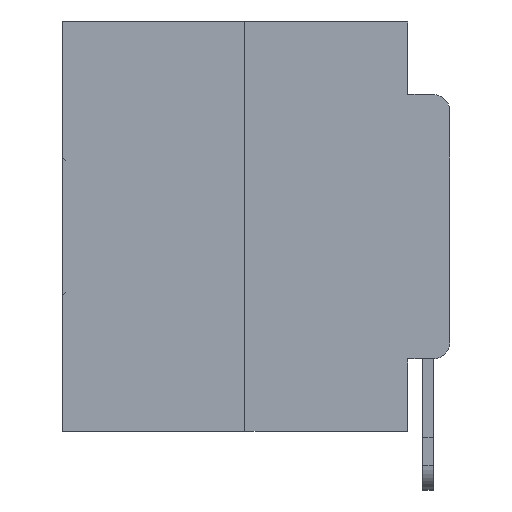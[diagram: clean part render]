
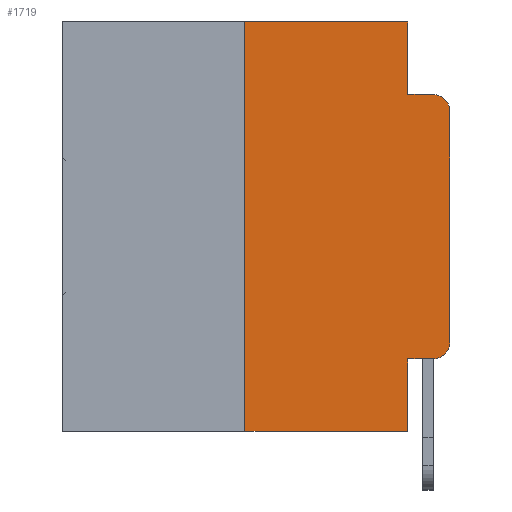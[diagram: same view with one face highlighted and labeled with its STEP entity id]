
A CAD part, left-side view. The second image highlights one B-rep face of the part: STEP entity #1719.
In plain terms, the highlighted planar face has unit normal (-1, 0, 0).
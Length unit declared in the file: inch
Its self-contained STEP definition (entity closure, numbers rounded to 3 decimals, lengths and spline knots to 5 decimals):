
#483 = VERTEX_POINT ( 'NONE', #22196 ) ;
#637 = EDGE_CURVE ( 'NONE', #29164, #14977, #27600, .T. ) ;
#1609 = LINE ( 'NONE', #19045, #25815 ) ;
#1719 = ADVANCED_FACE ( 'NONE', ( #14813 ), #16673, .F. ) ;
#2117 = VERTEX_POINT ( 'NONE', #26497 ) ;
#2672 = CARTESIAN_POINT ( 'NONE',  ( 0., 0.051, -0.4115 ) ) ;
#2857 = VECTOR ( 'NONE', #12735, 39.37008 ) ;
#3041 = LINE ( 'NONE', #29025, #21032 ) ;
#4005 = CARTESIAN_POINT ( 'NONE',  ( 0., 0.02, -0.3915 ) ) ;
#4064 = EDGE_CURVE ( 'NONE', #19747, #24746, #23644, .T. ) ;
#4515 = CARTESIAN_POINT ( 'NONE',  ( 0., 0.25, -0.5 ) ) ;
#5042 = VECTOR ( 'NONE', #19526, 39.37008 ) ;
#5361 = EDGE_CURVE ( 'NONE', #24746, #19540, #11165, .T. ) ;
#5516 = CARTESIAN_POINT ( 'NONE',  ( 0., 0.25, 0. ) ) ;
#6469 = DIRECTION ( 'NONE',  ( 0., 0., -1. ) ) ;
#7236 = ORIENTED_EDGE ( 'NONE', *, *, #29345, .T. ) ;
#7372 = EDGE_CURVE ( 'NONE', #19540, #11753, #22399, .T. ) ;
#7907 = CARTESIAN_POINT ( 'NONE',  ( 0., 0., 0. ) ) ;
#8372 = CARTESIAN_POINT ( 'NONE',  ( 0., 0.051, -0.4115 ) ) ;
#8874 = AXIS2_PLACEMENT_3D ( 'NONE', #4005, #20400, #6469 ) ;
#9543 = LINE ( 'NONE', #8372, #14988 ) ;
#10212 = VERTEX_POINT ( 'NONE', #30005 ) ;
#10434 = DIRECTION ( 'NONE',  ( -1., 0., 0. ) ) ;
#10787 = VERTEX_POINT ( 'NONE', #30152 ) ;
#10940 = DIRECTION ( 'NONE',  ( 0., -1., 0. ) ) ;
#11165 = LINE ( 'NONE', #28586, #22583 ) ;
#11355 = ORIENTED_EDGE ( 'NONE', *, *, #24942, .T. ) ;
#11723 = CARTESIAN_POINT ( 'NONE',  ( 0., 0.051, 0. ) ) ;
#11751 = DIRECTION ( 'NONE',  ( 0., -1., 0. ) ) ;
#11753 = VERTEX_POINT ( 'NONE', #28512 ) ;
#12009 = AXIS2_PLACEMENT_3D ( 'NONE', #16649, #13700, #16009 ) ;
#12094 = ORIENTED_EDGE ( 'NONE', *, *, #7372, .F. ) ;
#12182 = EDGE_CURVE ( 'NONE', #11753, #2117, #1609, .T. ) ;
#12297 = DIRECTION ( 'NONE',  ( 0., -1., 0. ) ) ;
#12355 = EDGE_LOOP ( 'NONE', ( #22038, #28023, #23506, #12094, #18129, #25594, #15638, #29026, #7236, #11355 ) ) ;
#12606 = CARTESIAN_POINT ( 'NONE',  ( 0., 0.051, 0. ) ) ;
#12686 = CIRCLE ( 'NONE', #23749, 0.02 ) ;
#12735 = DIRECTION ( 'NONE',  ( 0., 0., -1. ) ) ;
#13700 = DIRECTION ( 'NONE',  ( 1., 0., 0. ) ) ;
#13731 = EDGE_CURVE ( 'NONE', #483, #2117, #12686, .T. ) ;
#14813 = FACE_OUTER_BOUND ( 'NONE', #12355, .T. ) ;
#14977 = VERTEX_POINT ( 'NONE', #21245 ) ;
#14988 = VECTOR ( 'NONE', #26692, 39.37008 ) ;
#15625 = VECTOR ( 'NONE', #28400, 39.37008 ) ;
#15638 = ORIENTED_EDGE ( 'NONE', *, *, #19053, .T. ) ;
#15677 = VECTOR ( 'NONE', #21703, 39.37008 ) ;
#16009 = DIRECTION ( 'NONE',  ( 0., 0., -1. ) ) ;
#16649 = CARTESIAN_POINT ( 'NONE',  ( 0., 0.473, 0. ) ) ;
#16673 = PLANE ( 'NONE',  #12009 ) ;
#16748 = EDGE_CURVE ( 'NONE', #10787, #483, #27726, .T. ) ;
#18129 = ORIENTED_EDGE ( 'NONE', *, *, #5361, .F. ) ;
#19045 = CARTESIAN_POINT ( 'NONE',  ( 0., 0.051, -0.0885 ) ) ;
#19053 = EDGE_CURVE ( 'NONE', #19747, #14977, #3041, .T. ) ;
#19192 = CARTESIAN_POINT ( 'NONE',  ( 0., 0.25, 0. ) ) ;
#19526 = DIRECTION ( 'NONE',  ( 0., 0., 1. ) ) ;
#19540 = VERTEX_POINT ( 'NONE', #20184 ) ;
#19747 = VERTEX_POINT ( 'NONE', #4515 ) ;
#20184 = CARTESIAN_POINT ( 'NONE',  ( 0., 0.051, 0. ) ) ;
#20400 = DIRECTION ( 'NONE',  ( -1., 0., 0. ) ) ;
#21032 = VECTOR ( 'NONE', #10940, 39.37008 ) ;
#21245 = CARTESIAN_POINT ( 'NONE',  ( 0., 0.051, -0.5 ) ) ;
#21703 = DIRECTION ( 'NONE',  ( 0., 0., 1. ) ) ;
#22038 = ORIENTED_EDGE ( 'NONE', *, *, #16748, .T. ) ;
#22196 = CARTESIAN_POINT ( 'NONE',  ( 0., 0., -0.1085 ) ) ;
#22399 = LINE ( 'NONE', #12606, #15625 ) ;
#22583 = VECTOR ( 'NONE', #11751, 39.37008 ) ;
#23506 = ORIENTED_EDGE ( 'NONE', *, *, #12182, .F. ) ;
#23644 = LINE ( 'NONE', #19192, #5042 ) ;
#23749 = AXIS2_PLACEMENT_3D ( 'NONE', #24120, #10434, #26334 ) ;
#24120 = CARTESIAN_POINT ( 'NONE',  ( 0., 0.02, -0.1085 ) ) ;
#24746 = VERTEX_POINT ( 'NONE', #5516 ) ;
#24942 = EDGE_CURVE ( 'NONE', #10212, #10787, #28914, .T. ) ;
#25594 = ORIENTED_EDGE ( 'NONE', *, *, #4064, .F. ) ;
#25815 = VECTOR ( 'NONE', #12297, 39.37008 ) ;
#26334 = DIRECTION ( 'NONE',  ( 0., 0., -1. ) ) ;
#26497 = CARTESIAN_POINT ( 'NONE',  ( 0., 0.02, -0.0885 ) ) ;
#26692 = DIRECTION ( 'NONE',  ( 0., -1., 0. ) ) ;
#27600 = LINE ( 'NONE', #11723, #2857 ) ;
#27726 = LINE ( 'NONE', #7907, #15677 ) ;
#28023 = ORIENTED_EDGE ( 'NONE', *, *, #13731, .T. ) ;
#28400 = DIRECTION ( 'NONE',  ( 0., 0., -1. ) ) ;
#28512 = CARTESIAN_POINT ( 'NONE',  ( 0., 0.051, -0.0885 ) ) ;
#28586 = CARTESIAN_POINT ( 'NONE',  ( 0., 0.473, 0. ) ) ;
#28914 = CIRCLE ( 'NONE', #8874, 0.02 ) ;
#29025 = CARTESIAN_POINT ( 'NONE',  ( 0., 0.473, -0.5 ) ) ;
#29026 = ORIENTED_EDGE ( 'NONE', *, *, #637, .F. ) ;
#29164 = VERTEX_POINT ( 'NONE', #2672 ) ;
#29345 = EDGE_CURVE ( 'NONE', #29164, #10212, #9543, .T. ) ;
#30005 = CARTESIAN_POINT ( 'NONE',  ( 0., 0.02, -0.4115 ) ) ;
#30152 = CARTESIAN_POINT ( 'NONE',  ( 0., 0., -0.3915 ) ) ;
